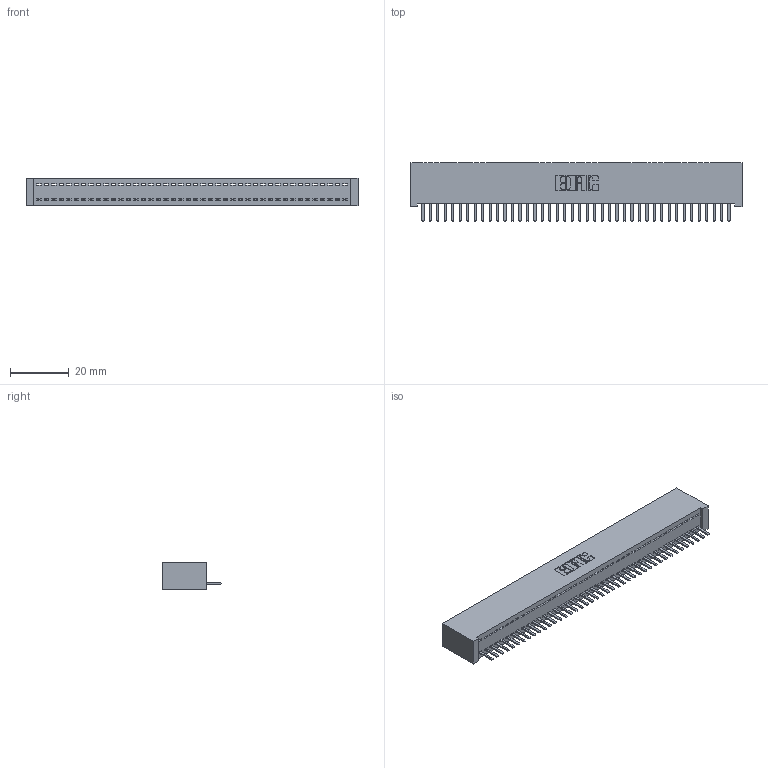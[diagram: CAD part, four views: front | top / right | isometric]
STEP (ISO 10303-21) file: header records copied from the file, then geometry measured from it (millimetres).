
FILE_DESCRIPTION (( 'STEP AP203' ), '1' );
FILE_NAME ('342-042-520-101.STEP', '2018-08-12T02:11:37', ( '' ), ( '' ), 'SwSTEP 2.0', 'SolidWorks 2016', '' );
FILE_SCHEMA (( 'CONFIG_CONTROL_DESIGN' ));
Length unit declared in the file: inch
Products named in the file (3): 342-042-520-101; 342 Part_Lugless; 345-292-001_345-293-120
Assembly tree (43 placements, depth 2):
  342-042-520-101
    342 Part_Lugless
    345-292-001_345-293-120  x42
Bounding box: 112.93 x 20.02 x 9.4 mm (x, y, z)
Volume: 10189.7 mm3; surface area: 14900 mm2
Topology: 43 solids, 43 shells, 2706 faces, 8003 edges, 5222 vertices
Faces by surface type: plane 1910, cylinder 796
Entity records: 25381 total; most frequent: CARTESIAN_POINT 4396, ORIENTED_EDGE 4362, DIRECTION 3689, EDGE_CURVE 2181, LINE 2057, VECTOR 2057, VERTEX_POINT 1450, AXIS2_PLACEMENT_3D 816
